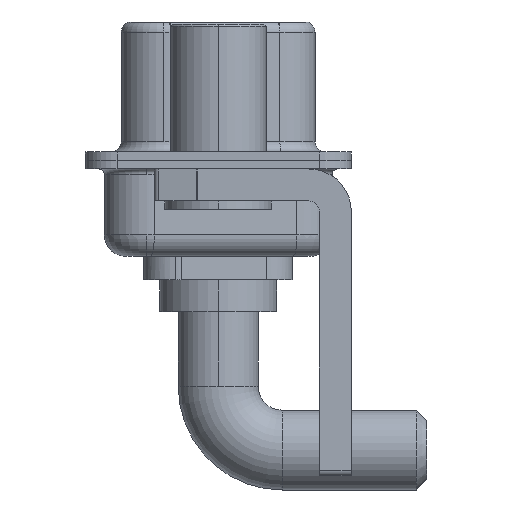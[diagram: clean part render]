
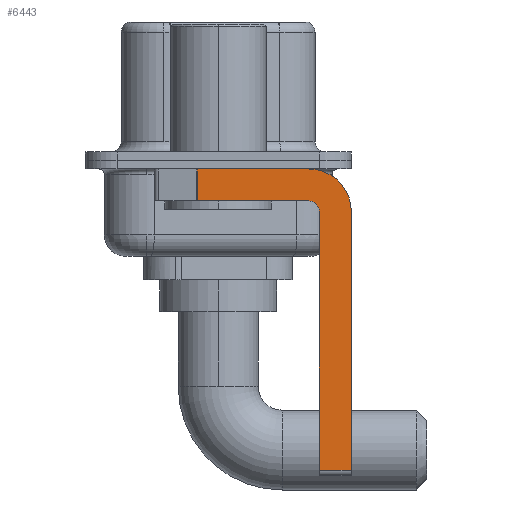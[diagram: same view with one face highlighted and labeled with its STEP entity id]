
A CAD part, left-side view. The second image highlights one B-rep face of the part: STEP entity #6443.
In plain terms, the highlighted planar face has unit normal (-1, 0, 0).
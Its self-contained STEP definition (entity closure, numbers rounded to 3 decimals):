
#222 = VECTOR ( 'NONE', #3733, 1000. ) ;
#294 = CARTESIAN_POINT ( 'NONE',  ( -2.9, 3., -0.4 ) ) ;
#395 = DIRECTION ( 'NONE',  ( 1., 0., 0. ) ) ;
#546 = ORIENTED_EDGE ( 'NONE', *, *, #8463, .F. ) ;
#941 = CARTESIAN_POINT ( 'NONE',  ( -2.9, 0.978, -0.4 ) ) ;
#971 = CARTESIAN_POINT ( 'NONE',  ( -2.9, -4.75, -14.8 ) ) ;
#1047 = VECTOR ( 'NONE', #18598, 1000. ) ;
#1108 = EDGE_CURVE ( 'NONE', #7531, #7703, #17091, .T. ) ;
#1809 = CARTESIAN_POINT ( 'NONE',  ( -2.9, -6.25, -14.55 ) ) ;
#1895 = ORIENTED_EDGE ( 'NONE', *, *, #18325, .T. ) ;
#1932 = DIRECTION ( 'NONE',  ( 1., 0., 0. ) ) ;
#2199 = EDGE_LOOP ( 'NONE', ( #3127, #1895, #546, #3940, #9704, #2722, #8491, #12024 ) ) ;
#2253 = CARTESIAN_POINT ( 'NONE',  ( -2.9, -4.25, -1.9 ) ) ;
#2722 = ORIENTED_EDGE ( 'NONE', *, *, #1108, .T. ) ;
#3010 = CARTESIAN_POINT ( 'NONE',  ( -2.9, -4.75, -2.4 ) ) ;
#3127 = ORIENTED_EDGE ( 'NONE', *, *, #12164, .F. ) ;
#3297 = PLANE ( 'NONE',  #5157 ) ;
#3733 = DIRECTION ( 'NONE',  ( 0., 0., -1. ) ) ;
#3793 = CARTESIAN_POINT ( 'NONE',  ( -2.9, -4.25, -1.9 ) ) ;
#3940 = ORIENTED_EDGE ( 'NONE', *, *, #8106, .F. ) ;
#4608 = VERTEX_POINT ( 'NONE', #941 ) ;
#5054 = VERTEX_POINT ( 'NONE', #16354 ) ;
#5157 = AXIS2_PLACEMENT_3D ( 'NONE', #14882, #395, #13920 ) ;
#5750 = AXIS2_PLACEMENT_3D ( 'NONE', #14310, #11375, #13060 ) ;
#6443 = ADVANCED_FACE ( 'NONE', ( #14703 ), #3297, .F. ) ;
#6824 = VECTOR ( 'NONE', #13059, 1000. ) ;
#7048 = VECTOR ( 'NONE', #18200, 1000. ) ;
#7332 = CIRCLE ( 'NONE', #9142, 2. ) ;
#7507 = VERTEX_POINT ( 'NONE', #3793 ) ;
#7531 = VERTEX_POINT ( 'NONE', #9519 ) ;
#7597 = DIRECTION ( 'NONE',  ( 0., -1., 0. ) ) ;
#7703 = VERTEX_POINT ( 'NONE', #1809 ) ;
#8097 = LINE ( 'NONE', #971, #7048 ) ;
#8106 = EDGE_CURVE ( 'NONE', #14048, #7507, #17200, .T. ) ;
#8463 = EDGE_CURVE ( 'NONE', #7507, #13864, #11164, .T. ) ;
#8491 = ORIENTED_EDGE ( 'NONE', *, *, #15177, .F. ) ;
#9142 = AXIS2_PLACEMENT_3D ( 'NONE', #17565, #1932, #13406 ) ;
#9482 = VECTOR ( 'NONE', #7597, 1000. ) ;
#9519 = CARTESIAN_POINT ( 'NONE',  ( -2.9, -4.75, -14.55 ) ) ;
#9645 = LINE ( 'NONE', #13629, #222 ) ;
#9704 = ORIENTED_EDGE ( 'NONE', *, *, #11808, .F. ) ;
#9953 = VECTOR ( 'NONE', #14014, 1000. ) ;
#11164 = LINE ( 'NONE', #2253, #9953 ) ;
#11329 = EDGE_CURVE ( 'NONE', #5054, #14711, #7332, .T. ) ;
#11375 = DIRECTION ( 'NONE',  ( -1., 0., 0. ) ) ;
#11808 = EDGE_CURVE ( 'NONE', #7531, #14048, #8097, .T. ) ;
#12024 = ORIENTED_EDGE ( 'NONE', *, *, #11329, .F. ) ;
#12164 = EDGE_CURVE ( 'NONE', #4608, #5054, #14779, .T. ) ;
#12836 = CARTESIAN_POINT ( 'NONE',  ( -2.9, -4.25, -14.55 ) ) ;
#13059 = DIRECTION ( 'NONE',  ( 0., 0., -1. ) ) ;
#13060 = DIRECTION ( 'NONE',  ( 0., 0., 1. ) ) ;
#13406 = DIRECTION ( 'NONE',  ( 0., 0., -1. ) ) ;
#13629 = CARTESIAN_POINT ( 'NONE',  ( -2.9, -6.25, -2.4 ) ) ;
#13864 = VERTEX_POINT ( 'NONE', #16153 ) ;
#13920 = DIRECTION ( 'NONE',  ( 0., 0., -1. ) ) ;
#14014 = DIRECTION ( 'NONE',  ( 0., 1., 0. ) ) ;
#14048 = VERTEX_POINT ( 'NONE', #3010 ) ;
#14218 = LINE ( 'NONE', #18552, #6824 ) ;
#14310 = CARTESIAN_POINT ( 'NONE',  ( -2.9, -4.25, -2.4 ) ) ;
#14703 = FACE_OUTER_BOUND ( 'NONE', #2199, .T. ) ;
#14711 = VERTEX_POINT ( 'NONE', #18617 ) ;
#14779 = LINE ( 'NONE', #294, #9482 ) ;
#14882 = CARTESIAN_POINT ( 'NONE',  ( -2.9, -4.25, -2.4 ) ) ;
#15177 = EDGE_CURVE ( 'NONE', #14711, #7703, #9645, .T. ) ;
#16153 = CARTESIAN_POINT ( 'NONE',  ( -2.9, 0.978, -1.9 ) ) ;
#16354 = CARTESIAN_POINT ( 'NONE',  ( -2.9, -4.25, -0.4 ) ) ;
#17091 = LINE ( 'NONE', #12836, #1047 ) ;
#17200 = CIRCLE ( 'NONE', #5750, 0.5 ) ;
#17565 = CARTESIAN_POINT ( 'NONE',  ( -2.9, -4.25, -2.4 ) ) ;
#18200 = DIRECTION ( 'NONE',  ( 0., 0., 1. ) ) ;
#18325 = EDGE_CURVE ( 'NONE', #4608, #13864, #14218, .T. ) ;
#18552 = CARTESIAN_POINT ( 'NONE',  ( -2.9, 0.978, -1.9 ) ) ;
#18598 = DIRECTION ( 'NONE',  ( 0., -1., 0. ) ) ;
#18617 = CARTESIAN_POINT ( 'NONE',  ( -2.9, -6.25, -2.4 ) ) ;
